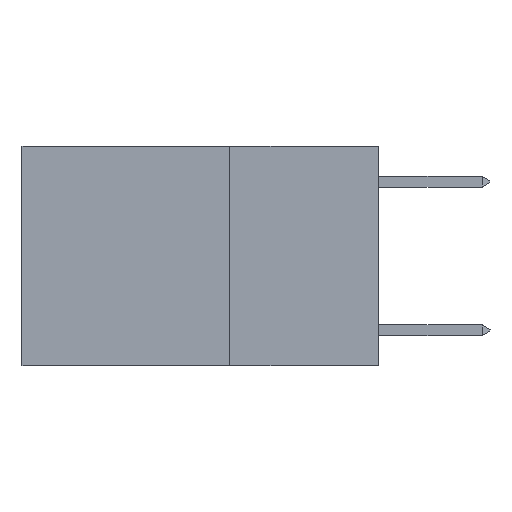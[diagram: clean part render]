
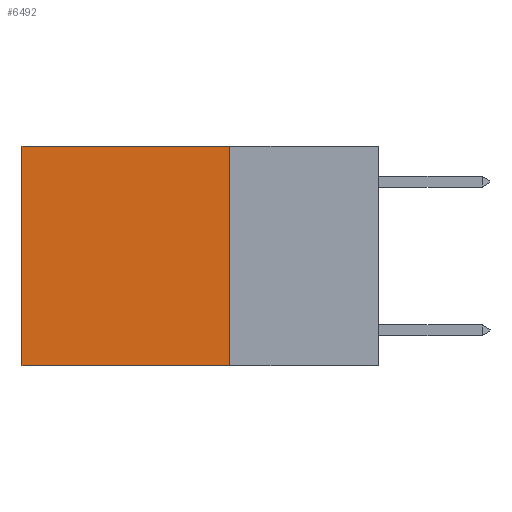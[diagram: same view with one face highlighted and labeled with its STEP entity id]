
A CAD part, left-side view. The second image highlights one B-rep face of the part: STEP entity #6492.
In plain terms, the highlighted planar face has unit normal (-1, 0, 0).
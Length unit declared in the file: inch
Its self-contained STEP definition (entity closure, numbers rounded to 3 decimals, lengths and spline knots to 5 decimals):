
#349 = DIRECTION ( 'NONE',  ( 0., 1., 0. ) ) ;
#1010 = DIRECTION ( 'NONE',  ( 0., 0., -1. ) ) ;
#1622 = CARTESIAN_POINT ( 'NONE',  ( 0.2625, 0.6, -0.37 ) ) ;
#2430 = ORIENTED_EDGE ( 'NONE', *, *, #6731, .T. ) ;
#3067 = VECTOR ( 'NONE', #4820, 39.37008 ) ;
#3255 = CARTESIAN_POINT ( 'NONE',  ( 0.2625, 0.25, 0. ) ) ;
#4820 = DIRECTION ( 'NONE',  ( 0., 0., -1. ) ) ;
#5125 = DIRECTION ( 'NONE',  ( 1., 0., 0. ) ) ;
#5664 = VECTOR ( 'NONE', #1010, 39.37008 ) ;
#5798 = CARTESIAN_POINT ( 'NONE',  ( 0.2625, 0.25, -0.37 ) ) ;
#5934 = AXIS2_PLACEMENT_3D ( 'NONE', #18820, #5125, #15890 ) ;
#6232 = EDGE_CURVE ( 'NONE', #15951, #9199, #11258, .T. ) ;
#6492 = ADVANCED_FACE ( 'NONE', ( #10523 ), #6626, .F. ) ;
#6626 = PLANE ( 'NONE',  #5934 ) ;
#6731 = EDGE_CURVE ( 'NONE', #13099, #9199, #9777, .T. ) ;
#7642 = VECTOR ( 'NONE', #15024, 39.37008 ) ;
#7650 = VECTOR ( 'NONE', #349, 39.37008 ) ;
#8302 = CARTESIAN_POINT ( 'NONE',  ( 0.2625, 0.6, 0. ) ) ;
#9199 = VERTEX_POINT ( 'NONE', #1622 ) ;
#9685 = VERTEX_POINT ( 'NONE', #13542 ) ;
#9777 = LINE ( 'NONE', #16420, #5664 ) ;
#10523 = FACE_OUTER_BOUND ( 'NONE', #13039, .T. ) ;
#11258 = LINE ( 'NONE', #5798, #7642 ) ;
#11329 = ORIENTED_EDGE ( 'NONE', *, *, #16599, .T. ) ;
#11644 = ORIENTED_EDGE ( 'NONE', *, *, #6232, .F. ) ;
#11782 = LINE ( 'NONE', #3255, #3067 ) ;
#12255 = LINE ( 'NONE', #18793, #7650 ) ;
#13039 = EDGE_LOOP ( 'NONE', ( #2430, #11644, #16388, #11329 ) ) ;
#13099 = VERTEX_POINT ( 'NONE', #8302 ) ;
#13542 = CARTESIAN_POINT ( 'NONE',  ( 0.2625, 0.25, 0. ) ) ;
#15024 = DIRECTION ( 'NONE',  ( 0., 1., 0. ) ) ;
#15032 = EDGE_CURVE ( 'NONE', #9685, #15951, #11782, .T. ) ;
#15890 = DIRECTION ( 'NONE',  ( 0., 0., -1. ) ) ;
#15951 = VERTEX_POINT ( 'NONE', #19152 ) ;
#16388 = ORIENTED_EDGE ( 'NONE', *, *, #15032, .F. ) ;
#16420 = CARTESIAN_POINT ( 'NONE',  ( 0.2625, 0.6, 0. ) ) ;
#16599 = EDGE_CURVE ( 'NONE', #9685, #13099, #12255, .T. ) ;
#18793 = CARTESIAN_POINT ( 'NONE',  ( 0.2625, 0.25, 0. ) ) ;
#18820 = CARTESIAN_POINT ( 'NONE',  ( 0.2625, 0.25, 0. ) ) ;
#19152 = CARTESIAN_POINT ( 'NONE',  ( 0.2625, 0.25, -0.37 ) ) ;
